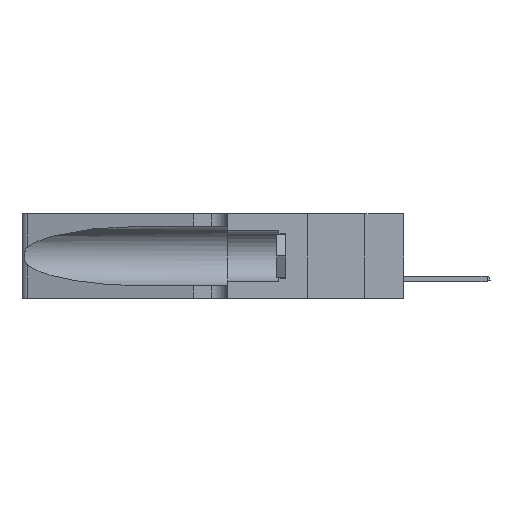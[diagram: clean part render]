
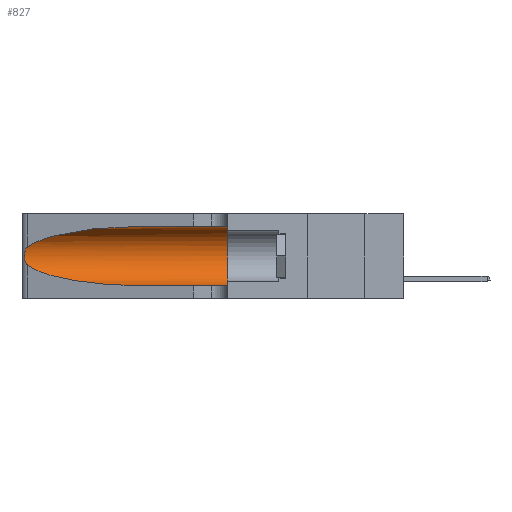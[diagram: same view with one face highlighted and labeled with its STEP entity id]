
A CAD part, left-side view. The second image highlights one B-rep face of the part: STEP entity #827.
In plain terms, the highlighted cylindrical face has radius 3.308 mm (diameter 6.617 mm), a partial arc.
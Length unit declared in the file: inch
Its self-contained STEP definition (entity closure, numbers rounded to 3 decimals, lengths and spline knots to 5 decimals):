
#5 = CARTESIAN_POINT ( 'NONE',  ( 0.25487, 1.22718, 0.14631 ) ) ;
#70 = ORIENTED_EDGE ( 'NONE', *, *, #25122, .T. ) ;
#827 = ADVANCED_FACE ( 'NONE', ( #12325 ), #36951, .F. ) ;
#867 = EDGE_CURVE ( 'NONE', #37369, #32363, #35384, .T. ) ;
#1034 = CARTESIAN_POINT ( 'NONE',  ( 0.25487, 1.22718, 0.22369 ) ) ;
#1389 = ORIENTED_EDGE ( 'NONE', *, *, #12878, .T. ) ;
#2081 = CARTESIAN_POINT ( 'NONE',  ( 0.25639, 1.23184, 0.21858 ) ) ;
#2220 = CARTESIAN_POINT ( 'NONE',  ( 0.26018, 1.23835, 0.19895 ) ) ;
#2262 = CARTESIAN_POINT ( 'NONE',  ( 0.18966, 0.96281, 0.31525 ) ) ;
#2651 = CIRCLE ( 'NONE', #22872, 0.13025 ) ;
#3909 = CARTESIAN_POINT ( 'NONE',  ( 0.1305, 0.35, 0.05475 ) ) ;
#4309 =( BOUNDED_CURVE ( )  B_SPLINE_CURVE ( 3, ( #18214, #2262, #40314, #6811 ),
 .UNSPECIFIED., .F., .F. ) 
 B_SPLINE_CURVE_WITH_KNOTS ( ( 4, 4 ),
 ( 1.5708, 2.84003 ),
 .UNSPECIFIED. ) 
 CURVE ( )  GEOMETRIC_REPRESENTATION_ITEM ( )  RATIONAL_B_SPLINE_CURVE ( ( 1., 0.87, 0.87, 1. ) ) 
 REPRESENTATION_ITEM ( '' )  );
#4438 = DIRECTION ( 'NONE',  ( 0., 0., 1. ) ) ;
#5313 = VERTEX_POINT ( 'NONE', #16881 ) ;
#6561 = DIRECTION ( 'NONE',  ( 0., -1., 0. ) ) ;
#6746 = DIRECTION ( 'NONE',  ( 0., 0., -1. ) ) ;
#6802 =( BOUNDED_CURVE ( )  B_SPLINE_CURVE ( 3, ( #19632, #9567, #7058, #19231 ),
 .UNSPECIFIED., .F., .F. ) 
 B_SPLINE_CURVE_WITH_KNOTS ( ( 4, 4 ),
 ( 3.44316, 4.71239 ),
 .UNSPECIFIED. ) 
 CURVE ( )  GEOMETRIC_REPRESENTATION_ITEM ( )  RATIONAL_B_SPLINE_CURVE ( ( 1., 0.87, 0.87, 1. ) ) 
 REPRESENTATION_ITEM ( '' )  );
#6811 = CARTESIAN_POINT ( 'NONE',  ( 0.25487, 1.22718, 0.22369 ) ) ;
#7058 = CARTESIAN_POINT ( 'NONE',  ( 0.18966, 0.96281, 0.05475 ) ) ;
#8276 = VERTEX_POINT ( 'NONE', #35897 ) ;
#8513 = CARTESIAN_POINT ( 'NONE',  ( 0.26017, 1.23833, 0.17102 ) ) ;
#9567 = CARTESIAN_POINT ( 'NONE',  ( 0.2373, 1.15595, 0.08982 ) ) ;
#9598 = CARTESIAN_POINT ( 'NONE',  ( 0.1305, 1.61858, 0.31525 ) ) ;
#11307 = EDGE_CURVE ( 'NONE', #8276, #5313, #13790, .T. ) ;
#12325 = FACE_OUTER_BOUND ( 'NONE', #31003, .T. ) ;
#12452 = CARTESIAN_POINT ( 'NONE',  ( 0.1305, 1.61858, 0.185 ) ) ;
#12704 = VERTEX_POINT ( 'NONE', #27206 ) ;
#12878 = EDGE_CURVE ( 'NONE', #8276, #32357, #4309, .T. ) ;
#13790 = LINE ( 'NONE', #9598, #21220 ) ;
#14226 = CARTESIAN_POINT ( 'NONE',  ( 0.1305, 0.72297, 0.05475 ) ) ;
#14858 = CARTESIAN_POINT ( 'NONE',  ( 0.25789, 1.23486, 0.15765 ) ) ;
#15421 = CARTESIAN_POINT ( 'NONE',  ( 0.25639, 1.23186, 0.15144 ) ) ;
#15496 = EDGE_CURVE ( 'NONE', #5313, #32363, #2651, .T. ) ;
#15533 = ORIENTED_EDGE ( 'NONE', *, *, #15496, .F. ) ;
#16261 = CARTESIAN_POINT ( 'NONE',  ( 0.1305, 1.61858, 0.05475 ) ) ;
#16840 = CARTESIAN_POINT ( 'NONE',  ( 0.1305, 0.35, 0.185 ) ) ;
#16881 = CARTESIAN_POINT ( 'NONE',  ( 0.1305, 0.35, 0.31525 ) ) ;
#18214 = CARTESIAN_POINT ( 'NONE',  ( 0.1305, 0.72297, 0.31525 ) ) ;
#19231 = CARTESIAN_POINT ( 'NONE',  ( 0.1305, 0.72297, 0.05475 ) ) ;
#19632 = CARTESIAN_POINT ( 'NONE',  ( 0.25487, 1.22718, 0.14631 ) ) ;
#20224 = EDGE_CURVE ( 'NONE', #12704, #37369, #6802, .T. ) ;
#20826 = CARTESIAN_POINT ( 'NONE',  ( 0.25487, 1.22718, 0.22369 ) ) ;
#21220 = VECTOR ( 'NONE', #6561, 39.37008 ) ;
#22872 = AXIS2_PLACEMENT_3D ( 'NONE', #16840, #23213, #4438 ) ;
#23213 = DIRECTION ( 'NONE',  ( 0., 1., 0. ) ) ;
#24305 = CARTESIAN_POINT ( 'NONE',  ( 0.26075, 1.23896, 0.178 ) ) ;
#24451 = CARTESIAN_POINT ( 'NONE',  ( 0.25787, 1.23484, 0.2124 ) ) ;
#25122 = EDGE_CURVE ( 'NONE', #32357, #12704, #31784, .T. ) ;
#27155 = CARTESIAN_POINT ( 'NONE',  ( 0.25555, 1.22994, 0.2215 ) ) ;
#27206 = CARTESIAN_POINT ( 'NONE',  ( 0.25487, 1.22718, 0.14631 ) ) ;
#27561 = CARTESIAN_POINT ( 'NONE',  ( 0.26075, 1.23896, 0.19203 ) ) ;
#27975 = CARTESIAN_POINT ( 'NONE',  ( 0.25555, 1.22993, 0.14849 ) ) ;
#29009 = AXIS2_PLACEMENT_3D ( 'NONE', #12452, #32068, #6746 ) ;
#30537 = CARTESIAN_POINT ( 'NONE',  ( 0.25856, 1.23593, 0.16098 ) ) ;
#30998 = DIRECTION ( 'NONE',  ( 0., -1., 0. ) ) ;
#31003 = EDGE_LOOP ( 'NONE', ( #1389, #70, #38802, #31111, #15533, #36738 ) ) ;
#31111 = ORIENTED_EDGE ( 'NONE', *, *, #867, .T. ) ;
#31784 = B_SPLINE_CURVE_WITH_KNOTS ( 'NONE', 3,
 ( #20826, #27155, #2081, #24451, #39855, #2220, #27561, #24305, #8513, #30537, #14858, #15421, #27975, #5 ),
 .UNSPECIFIED., .F., .F.,
 ( 4, 2, 2, 2, 2, 2, 4 ),
 ( 0., 0.00027, 0.00053, 0.00107, 0.0016, 0.00187, 0.00214 ),
 .UNSPECIFIED. ) ;
#32068 = DIRECTION ( 'NONE',  ( 0., -1., 0. ) ) ;
#32357 = VERTEX_POINT ( 'NONE', #1034 ) ;
#32363 = VERTEX_POINT ( 'NONE', #3909 ) ;
#35384 = LINE ( 'NONE', #16261, #37906 ) ;
#35897 = CARTESIAN_POINT ( 'NONE',  ( 0.1305, 0.72297, 0.31525 ) ) ;
#36738 = ORIENTED_EDGE ( 'NONE', *, *, #11307, .F. ) ;
#36951 = CYLINDRICAL_SURFACE ( 'NONE', #29009, 0.13025 ) ;
#37369 = VERTEX_POINT ( 'NONE', #14226 ) ;
#37906 = VECTOR ( 'NONE', #30998, 39.37008 ) ;
#38802 = ORIENTED_EDGE ( 'NONE', *, *, #20224, .T. ) ;
#39855 = CARTESIAN_POINT ( 'NONE',  ( 0.25854, 1.2359, 0.20912 ) ) ;
#40314 = CARTESIAN_POINT ( 'NONE',  ( 0.2373, 1.15595, 0.28018 ) ) ;
